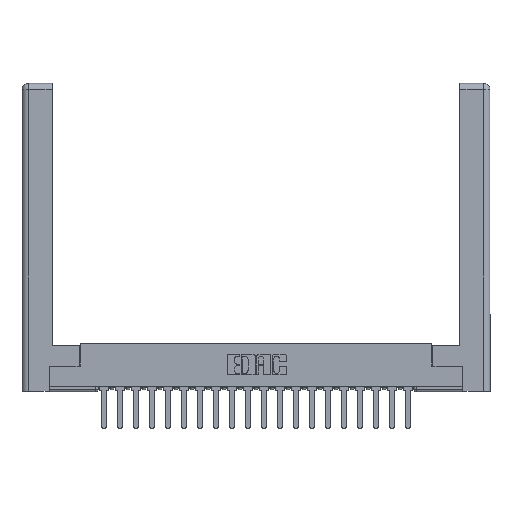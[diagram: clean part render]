
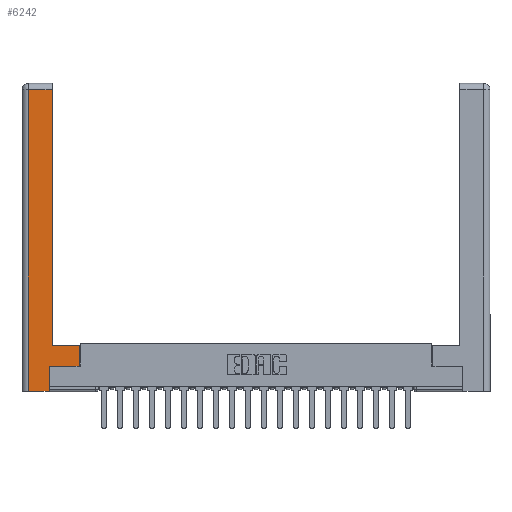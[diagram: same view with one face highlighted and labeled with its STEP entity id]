
A CAD part, top view. The second image highlights one B-rep face of the part: STEP entity #6242.
In plain terms, the highlighted planar face has unit normal (0, 0, 1).
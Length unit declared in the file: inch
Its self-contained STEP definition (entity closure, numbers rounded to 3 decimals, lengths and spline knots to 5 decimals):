
#173 = VECTOR ( 'NONE', #8965, 39.37008 ) ;
#679 = VECTOR ( 'NONE', #10312, 39.37008 ) ;
#773 = LINE ( 'NONE', #1002, #18013 ) ;
#1002 = CARTESIAN_POINT ( 'NONE',  ( 0.0615, 2.94, 0. ) ) ;
#1706 = DIRECTION ( 'NONE',  ( 0., 0., -1. ) ) ;
#1803 = DIRECTION ( 'NONE',  ( 1., 0., 0. ) ) ;
#2013 = EDGE_CURVE ( 'NONE', #20202, #12876, #17196, .T. ) ;
#2794 = EDGE_CURVE ( 'NONE', #7506, #11620, #773, .T. ) ;
#3305 = CARTESIAN_POINT ( 'NONE',  ( 0., 0., 0. ) ) ;
#3386 = CARTESIAN_POINT ( 'NONE',  ( 0.565, 0.45, 0. ) ) ;
#4952 = CARTESIAN_POINT ( 'NONE',  ( 0.295, 0.45, 0. ) ) ;
#5559 = ORIENTED_EDGE ( 'NONE', *, *, #21291, .T. ) ;
#6072 = VECTOR ( 'NONE', #12189, 39.37008 ) ;
#6242 = ADVANCED_FACE ( 'NONE', ( #13865 ), #18781, .F. ) ;
#6559 = CARTESIAN_POINT ( 'NONE',  ( 0.265, 0., 0. ) ) ;
#6594 = VECTOR ( 'NONE', #1803, 39.37008 ) ;
#6770 = CARTESIAN_POINT ( 'NONE',  ( 0.265, 0., 0. ) ) ;
#7252 = CARTESIAN_POINT ( 'NONE',  ( 0.0615, 0., 0. ) ) ;
#7506 = VERTEX_POINT ( 'NONE', #8683 ) ;
#7973 = DIRECTION ( 'NONE',  ( -1., 0., 0. ) ) ;
#7985 = VECTOR ( 'NONE', #13483, 39.37008 ) ;
#8342 = DIRECTION ( 'NONE',  ( 0., 1., 0. ) ) ;
#8683 = CARTESIAN_POINT ( 'NONE',  ( 0.295, 2.94, 0. ) ) ;
#8850 = ORIENTED_EDGE ( 'NONE', *, *, #2794, .T. ) ;
#8965 = DIRECTION ( 'NONE',  ( 0., -1., 0. ) ) ;
#9116 = CARTESIAN_POINT ( 'NONE',  ( 0.565, 0.245, 0. ) ) ;
#9485 = EDGE_CURVE ( 'NONE', #12876, #13692, #20786, .T. ) ;
#10275 = CARTESIAN_POINT ( 'NONE',  ( 0.265, 0.245, 0. ) ) ;
#10312 = DIRECTION ( 'NONE',  ( -1., 0., 0. ) ) ;
#11141 = EDGE_CURVE ( 'NONE', #13692, #13903, #20763, .T. ) ;
#11620 = VERTEX_POINT ( 'NONE', #20631 ) ;
#12189 = DIRECTION ( 'NONE',  ( 0., 1., 0. ) ) ;
#12386 = ORIENTED_EDGE ( 'NONE', *, *, #2013, .T. ) ;
#12460 = LINE ( 'NONE', #7252, #173 ) ;
#12499 = EDGE_CURVE ( 'NONE', #21573, #7506, #13539, .T. ) ;
#12876 = VERTEX_POINT ( 'NONE', #21097 ) ;
#12964 = CARTESIAN_POINT ( 'NONE',  ( 0.565, 0.45, 0. ) ) ;
#13264 = ORIENTED_EDGE ( 'NONE', *, *, #9485, .T. ) ;
#13437 = ORIENTED_EDGE ( 'NONE', *, *, #15806, .T. ) ;
#13483 = DIRECTION ( 'NONE',  ( 1., 0., 0. ) ) ;
#13539 = LINE ( 'NONE', #20575, #19191 ) ;
#13641 = CARTESIAN_POINT ( 'NONE',  ( 0.565, 0.245, 0. ) ) ;
#13692 = VERTEX_POINT ( 'NONE', #9116 ) ;
#13865 = FACE_OUTER_BOUND ( 'NONE', #19347, .T. ) ;
#13903 = VERTEX_POINT ( 'NONE', #12964 ) ;
#14562 = VECTOR ( 'NONE', #15650, 39.37008 ) ;
#14863 = ORIENTED_EDGE ( 'NONE', *, *, #11141, .T. ) ;
#15191 = LINE ( 'NONE', #4952, #679 ) ;
#15650 = DIRECTION ( 'NONE',  ( 0., 1., 0. ) ) ;
#15806 = EDGE_CURVE ( 'NONE', #11620, #17450, #12460, .T. ) ;
#16710 = ORIENTED_EDGE ( 'NONE', *, *, #21229, .T. ) ;
#16801 = ORIENTED_EDGE ( 'NONE', *, *, #12499, .T. ) ;
#16956 = DIRECTION ( 'NONE',  ( -1., 0., 0. ) ) ;
#17135 = AXIS2_PLACEMENT_3D ( 'NONE', #3305, #1706, #16956 ) ;
#17196 = LINE ( 'NONE', #10275, #6072 ) ;
#17450 = VERTEX_POINT ( 'NONE', #19818 ) ;
#18013 = VECTOR ( 'NONE', #7973, 39.37008 ) ;
#18663 = CARTESIAN_POINT ( 'NONE',  ( 0.295, 0.45, 0. ) ) ;
#18781 = PLANE ( 'NONE',  #17135 ) ;
#19191 = VECTOR ( 'NONE', #8342, 39.37008 ) ;
#19347 = EDGE_LOOP ( 'NONE', ( #16801, #8850, #13437, #16710, #12386, #13264, #14863, #5559 ) ) ;
#19818 = CARTESIAN_POINT ( 'NONE',  ( 0.0615, 0., 0. ) ) ;
#20202 = VERTEX_POINT ( 'NONE', #6770 ) ;
#20575 = CARTESIAN_POINT ( 'NONE',  ( 0.295, 3., 0. ) ) ;
#20631 = CARTESIAN_POINT ( 'NONE',  ( 0.0615, 2.94, 0. ) ) ;
#20763 = LINE ( 'NONE', #3386, #14562 ) ;
#20786 = LINE ( 'NONE', #13641, #6594 ) ;
#21097 = CARTESIAN_POINT ( 'NONE',  ( 0.265, 0.245, 0. ) ) ;
#21229 = EDGE_CURVE ( 'NONE', #17450, #20202, #22107, .T. ) ;
#21291 = EDGE_CURVE ( 'NONE', #13903, #21573, #15191, .T. ) ;
#21573 = VERTEX_POINT ( 'NONE', #18663 ) ;
#22107 = LINE ( 'NONE', #6559, #7985 ) ;
